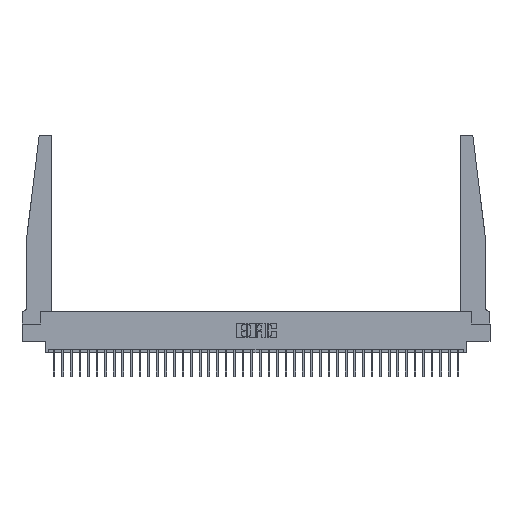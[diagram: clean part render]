
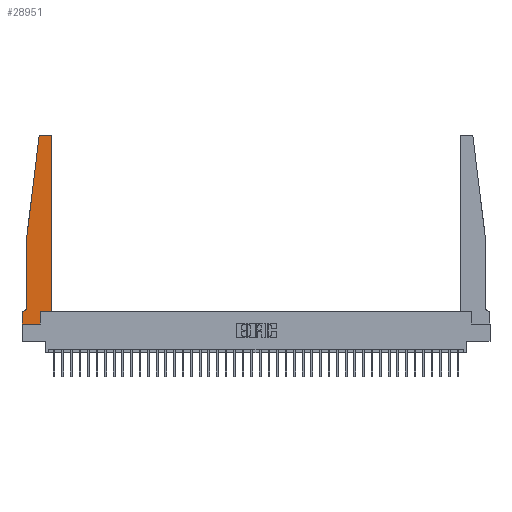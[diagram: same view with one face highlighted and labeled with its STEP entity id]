
A CAD part, top view. The second image highlights one B-rep face of the part: STEP entity #28951.
In plain terms, the highlighted planar face has unit normal (0, 0, 1).
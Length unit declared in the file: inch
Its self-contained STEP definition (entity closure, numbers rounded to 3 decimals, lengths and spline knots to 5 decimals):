
#521 = CARTESIAN_POINT ( 'NONE',  ( 0.395, 2.75, 0.37 ) ) ;
#599 = ORIENTED_EDGE ( 'NONE', *, *, #17169, .T. ) ;
#742 = ORIENTED_EDGE ( 'NONE', *, *, #34407, .T. ) ;
#1427 = LINE ( 'NONE', #7239, #21996 ) ;
#1706 = LINE ( 'NONE', #34631, #29707 ) ;
#2146 = DIRECTION ( 'NONE',  ( 0., 0., 1. ) ) ;
#2777 = VERTEX_POINT ( 'NONE', #521 ) ;
#3017 = DIRECTION ( 'NONE',  ( -1., 0., 0. ) ) ;
#3022 = CIRCLE ( 'NONE', #17000, 0.05 ) ;
#3169 = VERTEX_POINT ( 'NONE', #32692 ) ;
#3200 = CARTESIAN_POINT ( 'NONE',  ( 0., 0., 0.37 ) ) ;
#3243 = EDGE_CURVE ( 'NONE', #16038, #35517, #22513, .T. ) ;
#3465 = VERTEX_POINT ( 'NONE', #8571 ) ;
#3636 = AXIS2_PLACEMENT_3D ( 'NONE', #28361, #9259, #25642 ) ;
#3883 = VERTEX_POINT ( 'NONE', #16394 ) ;
#5096 = CARTESIAN_POINT ( 'NONE',  ( 0., 0., 0.37 ) ) ;
#5170 = VERTEX_POINT ( 'NONE', #5995 ) ;
#5271 = LINE ( 'NONE', #5096, #6983 ) ;
#5590 = VERTEX_POINT ( 'NONE', #13655 ) ;
#5875 = CARTESIAN_POINT ( 'NONE',  ( 0.2605, 0.18, 0.37 ) ) ;
#5995 = CARTESIAN_POINT ( 'NONE',  ( 0.2605, 0., 0.37 ) ) ;
#6107 = CARTESIAN_POINT ( 'NONE',  ( 0.25, 2.75, 0.37 ) ) ;
#6321 = CIRCLE ( 'NONE', #22621, 0.03 ) ;
#6705 = CARTESIAN_POINT ( 'NONE',  ( 0.015, 0.1875, 0.37 ) ) ;
#6795 = EDGE_CURVE ( 'NONE', #29236, #2777, #6321, .T. ) ;
#6810 = CARTESIAN_POINT ( 'NONE',  ( 0.425, 0.18, 0.37 ) ) ;
#6875 = VECTOR ( 'NONE', #3017, 39.37008 ) ;
#6983 = VECTOR ( 'NONE', #16399, 39.37008 ) ;
#7239 = CARTESIAN_POINT ( 'NONE',  ( 0.425, 0.18, 0.37 ) ) ;
#8483 = DIRECTION ( 'NONE',  ( -1., 0., 0. ) ) ;
#8571 = CARTESIAN_POINT ( 'NONE',  ( 0.065, 0.2375, 0.37 ) ) ;
#8683 = DIRECTION ( 'NONE',  ( -1., 0., 0. ) ) ;
#9259 = DIRECTION ( 'NONE',  ( 0., 0., 1. ) ) ;
#9741 = EDGE_CURVE ( 'NONE', #3465, #16038, #3022, .T. ) ;
#10448 = CARTESIAN_POINT ( 'NONE',  ( 0.425, 2.72, 0.37 ) ) ;
#10705 = CARTESIAN_POINT ( 'NONE',  ( 0.27653, 2.75, 0.37 ) ) ;
#11340 = EDGE_LOOP ( 'NONE', ( #14876, #19995, #12348, #25542, #20853, #22474, #742, #599, #23818, #27901, #26583, #27606 ) ) ;
#11489 = EDGE_CURVE ( 'NONE', #2777, #32174, #25058, .T. ) ;
#12348 = ORIENTED_EDGE ( 'NONE', *, *, #23156, .T. ) ;
#12544 = DIRECTION ( 'NONE',  ( 0., 1., 0. ) ) ;
#12759 = EDGE_CURVE ( 'NONE', #32174, #14990, #17093, .T. ) ;
#13096 = CARTESIAN_POINT ( 'NONE',  ( 0.27653, 2.72, 0.37 ) ) ;
#13655 = CARTESIAN_POINT ( 'NONE',  ( 0.2605, 0.18, 0.37 ) ) ;
#13914 = VECTOR ( 'NONE', #24841, 39.37008 ) ;
#14692 = CARTESIAN_POINT ( 'NONE',  ( 0.065, 0.1875, 0.37 ) ) ;
#14876 = ORIENTED_EDGE ( 'NONE', *, *, #11489, .T. ) ;
#14990 = VERTEX_POINT ( 'NONE', #23396 ) ;
#15019 = DIRECTION ( 'NONE',  ( 1., 0., 0. ) ) ;
#15233 = EDGE_CURVE ( 'NONE', #5170, #5590, #28089, .T. ) ;
#16038 = VERTEX_POINT ( 'NONE', #6705 ) ;
#16192 = DIRECTION ( 'NONE',  ( 0., -1., 0. ) ) ;
#16394 = CARTESIAN_POINT ( 'NONE',  ( 0., 0., 0.37 ) ) ;
#16399 = DIRECTION ( 'NONE',  ( 0., -1., 0. ) ) ;
#16863 = LINE ( 'NONE', #3200, #23756 ) ;
#17000 = AXIS2_PLACEMENT_3D ( 'NONE', #22539, #33596, #8683 ) ;
#17093 = CIRCLE ( 'NONE', #35101, 0.03 ) ;
#17169 = EDGE_CURVE ( 'NONE', #3883, #5170, #16863, .T. ) ;
#17906 = DIRECTION ( 'NONE',  ( -0.122, -0.992, 0. ) ) ;
#19092 = CARTESIAN_POINT ( 'NONE',  ( 0.065, 1.25, 0.37 ) ) ;
#19265 = DIRECTION ( 'NONE',  ( 0., 0., 1. ) ) ;
#19995 = ORIENTED_EDGE ( 'NONE', *, *, #12759, .T. ) ;
#20853 = ORIENTED_EDGE ( 'NONE', *, *, #9741, .T. ) ;
#21996 = VECTOR ( 'NONE', #12544, 39.37008 ) ;
#22191 = DIRECTION ( 'NONE',  ( 1., 0., 0. ) ) ;
#22474 = ORIENTED_EDGE ( 'NONE', *, *, #3243, .T. ) ;
#22513 = LINE ( 'NONE', #14692, #6875 ) ;
#22539 = CARTESIAN_POINT ( 'NONE',  ( 0.015, 0.2375, 0.37 ) ) ;
#22621 = AXIS2_PLACEMENT_3D ( 'NONE', #33068, #19265, #22191 ) ;
#23104 = FACE_OUTER_BOUND ( 'NONE', #11340, .T. ) ;
#23156 = EDGE_CURVE ( 'NONE', #14990, #3169, #1706, .T. ) ;
#23396 = CARTESIAN_POINT ( 'NONE',  ( 0.24675, 2.72367, 0.37 ) ) ;
#23756 = VECTOR ( 'NONE', #30854, 39.37008 ) ;
#23818 = ORIENTED_EDGE ( 'NONE', *, *, #15233, .T. ) ;
#24187 = DIRECTION ( 'NONE',  ( 1., 0., 0. ) ) ;
#24555 = VERTEX_POINT ( 'NONE', #26243 ) ;
#24841 = DIRECTION ( 'NONE',  ( 0., 1., 0. ) ) ;
#25058 = LINE ( 'NONE', #6107, #34425 ) ;
#25542 = ORIENTED_EDGE ( 'NONE', *, *, #31649, .T. ) ;
#25642 = DIRECTION ( 'NONE',  ( 1., 0., 0. ) ) ;
#25925 = LINE ( 'NONE', #6810, #31519 ) ;
#26026 = VECTOR ( 'NONE', #16192, 39.37008 ) ;
#26243 = CARTESIAN_POINT ( 'NONE',  ( 0.425, 0.18, 0.37 ) ) ;
#26583 = ORIENTED_EDGE ( 'NONE', *, *, #31845, .T. ) ;
#27083 = EDGE_CURVE ( 'NONE', #5590, #24555, #25925, .T. ) ;
#27606 = ORIENTED_EDGE ( 'NONE', *, *, #6795, .T. ) ;
#27901 = ORIENTED_EDGE ( 'NONE', *, *, #27083, .T. ) ;
#28089 = LINE ( 'NONE', #5875, #13914 ) ;
#28361 = CARTESIAN_POINT ( 'NONE',  ( 0., 0.1875, 0.37 ) ) ;
#28951 = ADVANCED_FACE ( 'NONE', ( #23104 ), #31082, .T. ) ;
#29236 = VERTEX_POINT ( 'NONE', #10448 ) ;
#29707 = VECTOR ( 'NONE', #17906, 39.37008 ) ;
#30017 = LINE ( 'NONE', #19092, #26026 ) ;
#30854 = DIRECTION ( 'NONE',  ( 1., 0., 0. ) ) ;
#31082 = PLANE ( 'NONE',  #3636 ) ;
#31519 = VECTOR ( 'NONE', #15019, 39.37008 ) ;
#31649 = EDGE_CURVE ( 'NONE', #3169, #3465, #30017, .T. ) ;
#31845 = EDGE_CURVE ( 'NONE', #24555, #29236, #1427, .T. ) ;
#32174 = VERTEX_POINT ( 'NONE', #10705 ) ;
#32692 = CARTESIAN_POINT ( 'NONE',  ( 0.065, 1.25, 0.37 ) ) ;
#33068 = CARTESIAN_POINT ( 'NONE',  ( 0.395, 2.72, 0.37 ) ) ;
#33596 = DIRECTION ( 'NONE',  ( 0., 0., -1. ) ) ;
#33849 = CARTESIAN_POINT ( 'NONE',  ( 0., 0.1875, 0.37 ) ) ;
#34407 = EDGE_CURVE ( 'NONE', #35517, #3883, #5271, .T. ) ;
#34425 = VECTOR ( 'NONE', #8483, 39.37008 ) ;
#34631 = CARTESIAN_POINT ( 'NONE',  ( 0.065, 1.25, 0.37 ) ) ;
#35101 = AXIS2_PLACEMENT_3D ( 'NONE', #13096, #2146, #24187 ) ;
#35517 = VERTEX_POINT ( 'NONE', #33849 ) ;
